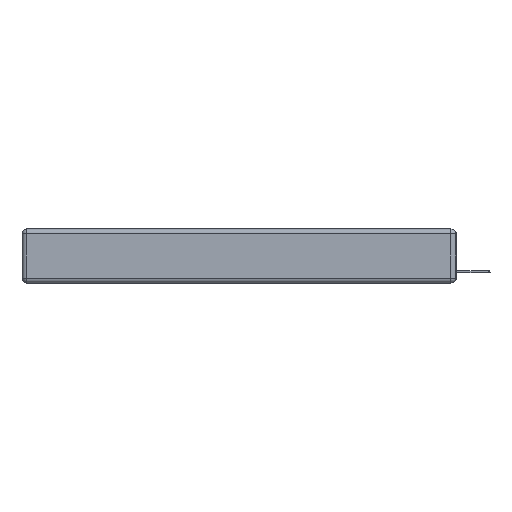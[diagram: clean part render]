
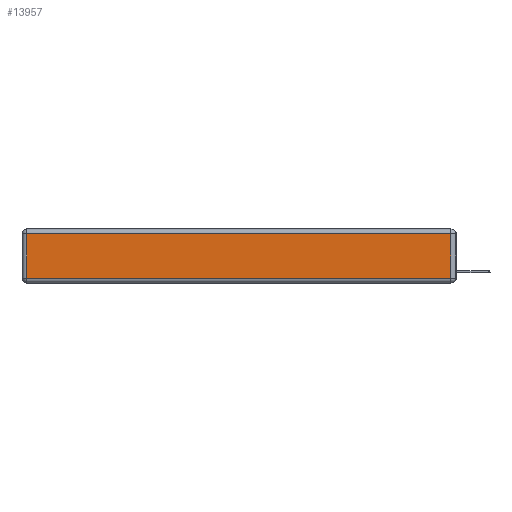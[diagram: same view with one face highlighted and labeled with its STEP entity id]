
A CAD part, left-side view. The second image highlights one B-rep face of the part: STEP entity #13957.
In plain terms, the highlighted planar face has unit normal (-1, 0, 0).
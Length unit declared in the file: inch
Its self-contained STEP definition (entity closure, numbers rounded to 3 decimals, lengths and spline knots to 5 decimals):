
#51 = ORIENTED_EDGE ( 'NONE', *, *, #1281, .T. ) ;
#54 = CARTESIAN_POINT ( 'NONE',  ( 0., 2.75, -0.03 ) ) ;
#1281 = EDGE_CURVE ( 'NONE', #5496, #13627, #1684, .T. ) ;
#1684 = LINE ( 'NONE', #14736, #4023 ) ;
#1727 = CARTESIAN_POINT ( 'NONE',  ( 0., 0.03, -0.343 ) ) ;
#1798 = VECTOR ( 'NONE', #6810, 39.37008 ) ;
#2160 = CARTESIAN_POINT ( 'NONE',  ( 0., 2.72, -0.313 ) ) ;
#2261 = FACE_OUTER_BOUND ( 'NONE', #5302, .T. ) ;
#2316 = DIRECTION ( 'NONE',  ( -1., 0., 0. ) ) ;
#3639 = DIRECTION ( 'NONE',  ( 0., -1., 0. ) ) ;
#3737 = DIRECTION ( 'NONE',  ( 0., 1., 0. ) ) ;
#3740 = EDGE_CURVE ( 'NONE', #12333, #5496, #4317, .T. ) ;
#4023 = VECTOR ( 'NONE', #3639, 39.37008 ) ;
#4317 = LINE ( 'NONE', #12959, #1798 ) ;
#4385 = VERTEX_POINT ( 'NONE', #5027 ) ;
#4976 = EDGE_CURVE ( 'NONE', #4385, #12333, #13077, .T. ) ;
#5027 = CARTESIAN_POINT ( 'NONE',  ( 0., 0.03, -0.03 ) ) ;
#5302 = EDGE_LOOP ( 'NONE', ( #51, #7460, #9080, #14175 ) ) ;
#5496 = VERTEX_POINT ( 'NONE', #2160 ) ;
#5893 = DIRECTION ( 'NONE',  ( 0., 0., 1. ) ) ;
#6810 = DIRECTION ( 'NONE',  ( 0., 0., -1. ) ) ;
#7460 = ORIENTED_EDGE ( 'NONE', *, *, #15671, .T. ) ;
#7699 = AXIS2_PLACEMENT_3D ( 'NONE', #13269, #2316, #5893 ) ;
#9080 = ORIENTED_EDGE ( 'NONE', *, *, #4976, .T. ) ;
#10470 = DIRECTION ( 'NONE',  ( 0., 0., 1. ) ) ;
#10755 = VECTOR ( 'NONE', #3737, 39.37008 ) ;
#11272 = CARTESIAN_POINT ( 'NONE',  ( 0., 0.03, -0.313 ) ) ;
#12000 = PLANE ( 'NONE',  #7699 ) ;
#12333 = VERTEX_POINT ( 'NONE', #15145 ) ;
#12959 = CARTESIAN_POINT ( 'NONE',  ( 0., 2.72, -0.343 ) ) ;
#13077 = LINE ( 'NONE', #54, #10755 ) ;
#13269 = CARTESIAN_POINT ( 'NONE',  ( 0., 0., -0.343 ) ) ;
#13627 = VERTEX_POINT ( 'NONE', #11272 ) ;
#13951 = VECTOR ( 'NONE', #10470, 39.37008 ) ;
#13957 = ADVANCED_FACE ( 'NONE', ( #2261 ), #12000, .T. ) ;
#14175 = ORIENTED_EDGE ( 'NONE', *, *, #3740, .T. ) ;
#14736 = CARTESIAN_POINT ( 'NONE',  ( 0., 0., -0.313 ) ) ;
#15104 = LINE ( 'NONE', #1727, #13951 ) ;
#15145 = CARTESIAN_POINT ( 'NONE',  ( 0., 2.72, -0.03 ) ) ;
#15671 = EDGE_CURVE ( 'NONE', #13627, #4385, #15104, .T. ) ;
